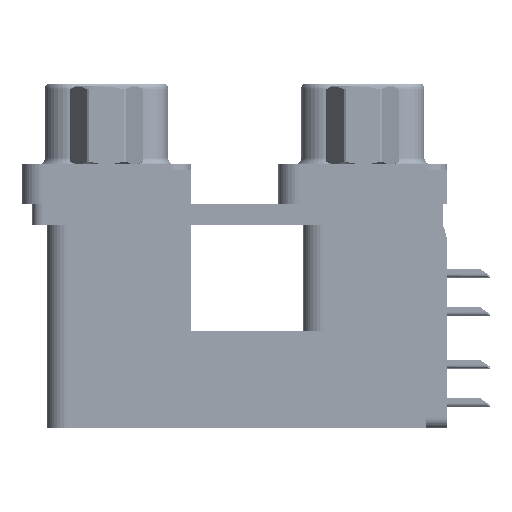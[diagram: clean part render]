
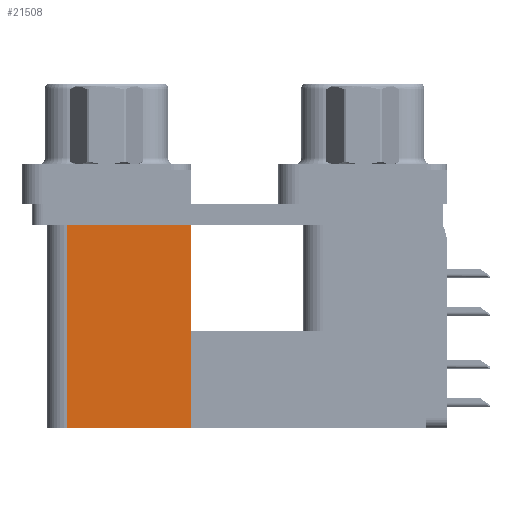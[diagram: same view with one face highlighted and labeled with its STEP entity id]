
A CAD part, left-side view. The second image highlights one B-rep face of the part: STEP entity #21508.
In plain terms, the highlighted planar face has unit normal (-1, 0, 0).
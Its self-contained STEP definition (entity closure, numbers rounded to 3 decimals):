
#395 = EDGE_CURVE ( 'NONE', #23993, #49447, #55039, .T. ) ;
#4103 = PLANE ( 'NONE',  #24790 ) ;
#4367 = CARTESIAN_POINT ( 'NONE',  ( 3.79, 12.775, -19.2 ) ) ;
#4738 = CARTESIAN_POINT ( 'NONE',  ( 3.79, 21.975, -2.5 ) ) ;
#6161 = VECTOR ( 'NONE', #23271, 1000. ) ;
#7191 = CARTESIAN_POINT ( 'NONE',  ( 3.79, 12.775, -19.2 ) ) ;
#7820 = LINE ( 'NONE', #4367, #16780 ) ;
#8851 = VERTEX_POINT ( 'NONE', #4738 ) ;
#9800 = LINE ( 'NONE', #28093, #39059 ) ;
#11829 = VERTEX_POINT ( 'NONE', #30722 ) ;
#12992 = ORIENTED_EDGE ( 'NONE', *, *, #54111, .T. ) ;
#13988 = EDGE_CURVE ( 'NONE', #49447, #8851, #14259, .T. ) ;
#14259 = LINE ( 'NONE', #27480, #6161 ) ;
#16780 = VECTOR ( 'NONE', #22096, 1000. ) ;
#20627 = ORIENTED_EDGE ( 'NONE', *, *, #395, .F. ) ;
#20749 = ORIENTED_EDGE ( 'NONE', *, *, #26371, .T. ) ;
#21289 = DIRECTION ( 'NONE',  ( 1., 0., 0. ) ) ;
#21508 = ADVANCED_FACE ( 'NONE', ( #29190 ), #4103, .F. ) ;
#22096 = DIRECTION ( 'NONE',  ( 0., 0., 1. ) ) ;
#23271 = DIRECTION ( 'NONE',  ( 0., 0., 1. ) ) ;
#23993 = VERTEX_POINT ( 'NONE', #26925 ) ;
#24790 = AXIS2_PLACEMENT_3D ( 'NONE', #38178, #21289, #30024 ) ;
#26371 = EDGE_CURVE ( 'NONE', #23993, #11829, #7820, .T. ) ;
#26925 = CARTESIAN_POINT ( 'NONE',  ( 3.79, 12.775, -19.2 ) ) ;
#26983 = DIRECTION ( 'NONE',  ( 0., 1., 0. ) ) ;
#27480 = CARTESIAN_POINT ( 'NONE',  ( 3.79, 21.975, -19.2 ) ) ;
#28093 = CARTESIAN_POINT ( 'NONE',  ( 3.79, 12.775, -2.5 ) ) ;
#29190 = FACE_OUTER_BOUND ( 'NONE', #42001, .T. ) ;
#30024 = DIRECTION ( 'NONE',  ( 0., 0., -1. ) ) ;
#30722 = CARTESIAN_POINT ( 'NONE',  ( 3.79, 12.775, -2.5 ) ) ;
#33095 = DIRECTION ( 'NONE',  ( 0., 1., 0. ) ) ;
#38178 = CARTESIAN_POINT ( 'NONE',  ( 3.79, 12.775, -19.2 ) ) ;
#39059 = VECTOR ( 'NONE', #26983, 1000. ) ;
#41442 = CARTESIAN_POINT ( 'NONE',  ( 3.79, 21.975, -19.2 ) ) ;
#42001 = EDGE_LOOP ( 'NONE', ( #12992, #42051, #20627, #20749 ) ) ;
#42051 = ORIENTED_EDGE ( 'NONE', *, *, #13988, .F. ) ;
#47725 = VECTOR ( 'NONE', #33095, 1000. ) ;
#49447 = VERTEX_POINT ( 'NONE', #41442 ) ;
#54111 = EDGE_CURVE ( 'NONE', #11829, #8851, #9800, .T. ) ;
#55039 = LINE ( 'NONE', #7191, #47725 ) ;
